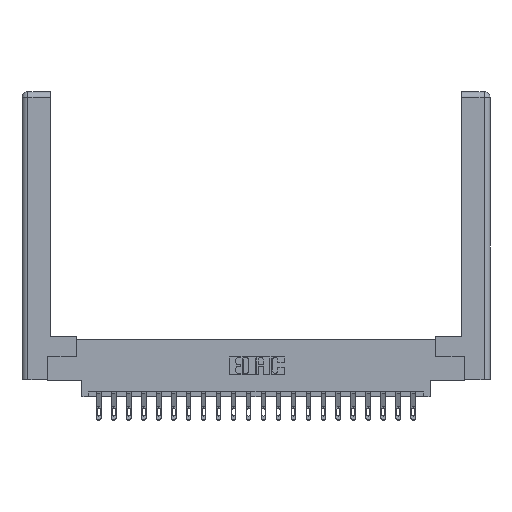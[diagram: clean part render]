
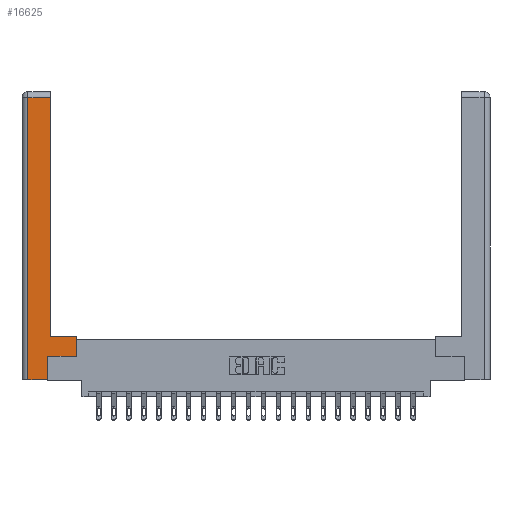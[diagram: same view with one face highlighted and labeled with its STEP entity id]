
A CAD part, top view. The second image highlights one B-rep face of the part: STEP entity #16625.
In plain terms, the highlighted planar face has unit normal (0, 0, 1).
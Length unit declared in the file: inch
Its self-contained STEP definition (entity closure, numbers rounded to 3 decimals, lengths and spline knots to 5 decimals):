
#794 = DIRECTION ( 'NONE',  ( 1., 0., 0. ) ) ;
#1180 = VERTEX_POINT ( 'NONE', #10161 ) ;
#1387 = CARTESIAN_POINT ( 'NONE',  ( 0.0615, 0., 0. ) ) ;
#1826 = VECTOR ( 'NONE', #3564, 39.37008 ) ;
#1943 = LINE ( 'NONE', #19112, #6294 ) ;
#2368 = CARTESIAN_POINT ( 'NONE',  ( 0.295, 2.94, 0. ) ) ;
#2577 = CARTESIAN_POINT ( 'NONE',  ( 0.265, 0., 0. ) ) ;
#2989 = VERTEX_POINT ( 'NONE', #10804 ) ;
#3122 = EDGE_CURVE ( 'NONE', #5500, #7006, #20719, .T. ) ;
#3294 = ORIENTED_EDGE ( 'NONE', *, *, #3122, .T. ) ;
#3403 = DIRECTION ( 'NONE',  ( 0., -1., 0. ) ) ;
#3490 = LINE ( 'NONE', #22546, #15811 ) ;
#3564 = DIRECTION ( 'NONE',  ( 1., 0., 0. ) ) ;
#3567 = CARTESIAN_POINT ( 'NONE',  ( 0., 0., 0. ) ) ;
#4233 = EDGE_CURVE ( 'NONE', #2989, #10051, #9920, .T. ) ;
#4491 = CARTESIAN_POINT ( 'NONE',  ( 0.265, 0.245, 0. ) ) ;
#4816 = LINE ( 'NONE', #18980, #5356 ) ;
#5103 = FACE_OUTER_BOUND ( 'NONE', #11005, .T. ) ;
#5356 = VECTOR ( 'NONE', #22328, 39.37008 ) ;
#5500 = VERTEX_POINT ( 'NONE', #2577 ) ;
#5528 = CARTESIAN_POINT ( 'NONE',  ( 0.565, 0.245, 0. ) ) ;
#5800 = VECTOR ( 'NONE', #9698, 39.37008 ) ;
#6276 = CARTESIAN_POINT ( 'NONE',  ( 0.565, 0.45, 0. ) ) ;
#6294 = VECTOR ( 'NONE', #3403, 39.37008 ) ;
#6546 = DIRECTION ( 'NONE',  ( -1., 0., 0. ) ) ;
#6777 = LINE ( 'NONE', #13402, #11740 ) ;
#6865 = EDGE_CURVE ( 'NONE', #11948, #5500, #20832, .T. ) ;
#7006 = VERTEX_POINT ( 'NONE', #4491 ) ;
#7509 = EDGE_CURVE ( 'NONE', #10051, #1180, #3490, .T. ) ;
#7518 = VECTOR ( 'NONE', #18393, 39.37008 ) ;
#8170 = EDGE_CURVE ( 'NONE', #1180, #8821, #4816, .T. ) ;
#8821 = VERTEX_POINT ( 'NONE', #2368 ) ;
#8831 = PLANE ( 'NONE',  #20022 ) ;
#9254 = ORIENTED_EDGE ( 'NONE', *, *, #15622, .T. ) ;
#9698 = DIRECTION ( 'NONE',  ( 0., 1., 0. ) ) ;
#9920 = LINE ( 'NONE', #11658, #5800 ) ;
#10051 = VERTEX_POINT ( 'NONE', #6276 ) ;
#10161 = CARTESIAN_POINT ( 'NONE',  ( 0.295, 0.45, 0. ) ) ;
#10804 = CARTESIAN_POINT ( 'NONE',  ( 0.565, 0.245, 0. ) ) ;
#11005 = EDGE_LOOP ( 'NONE', ( #16979, #11349, #17072, #18720, #3294, #9254, #19924, #19712 ) ) ;
#11349 = ORIENTED_EDGE ( 'NONE', *, *, #12863, .T. ) ;
#11658 = CARTESIAN_POINT ( 'NONE',  ( 0.565, 0.45, 0. ) ) ;
#11740 = VECTOR ( 'NONE', #6546, 39.37008 ) ;
#11948 = VERTEX_POINT ( 'NONE', #1387 ) ;
#12068 = VECTOR ( 'NONE', #794, 39.37008 ) ;
#12254 = DIRECTION ( 'NONE',  ( -1., 0., 0. ) ) ;
#12271 = VERTEX_POINT ( 'NONE', #17081 ) ;
#12849 = CARTESIAN_POINT ( 'NONE',  ( 0.265, 0., 0. ) ) ;
#12863 = EDGE_CURVE ( 'NONE', #8821, #12271, #6777, .T. ) ;
#13402 = CARTESIAN_POINT ( 'NONE',  ( 0.0615, 2.94, 0. ) ) ;
#15622 = EDGE_CURVE ( 'NONE', #7006, #2989, #22716, .T. ) ;
#15811 = VECTOR ( 'NONE', #12254, 39.37008 ) ;
#16625 = ADVANCED_FACE ( 'NONE', ( #5103 ), #8831, .F. ) ;
#16979 = ORIENTED_EDGE ( 'NONE', *, *, #8170, .T. ) ;
#17072 = ORIENTED_EDGE ( 'NONE', *, *, #21052, .T. ) ;
#17081 = CARTESIAN_POINT ( 'NONE',  ( 0.0615, 2.94, 0. ) ) ;
#18312 = CARTESIAN_POINT ( 'NONE',  ( 0.265, 0.245, 0. ) ) ;
#18393 = DIRECTION ( 'NONE',  ( 0., 1., 0. ) ) ;
#18720 = ORIENTED_EDGE ( 'NONE', *, *, #6865, .T. ) ;
#18980 = CARTESIAN_POINT ( 'NONE',  ( 0.295, 3., 0. ) ) ;
#19112 = CARTESIAN_POINT ( 'NONE',  ( 0.0615, 0., 0. ) ) ;
#19712 = ORIENTED_EDGE ( 'NONE', *, *, #7509, .T. ) ;
#19924 = ORIENTED_EDGE ( 'NONE', *, *, #4233, .T. ) ;
#20022 = AXIS2_PLACEMENT_3D ( 'NONE', #3567, #21144, #21068 ) ;
#20719 = LINE ( 'NONE', #18312, #7518 ) ;
#20832 = LINE ( 'NONE', #12849, #12068 ) ;
#21052 = EDGE_CURVE ( 'NONE', #12271, #11948, #1943, .T. ) ;
#21068 = DIRECTION ( 'NONE',  ( -1., 0., 0. ) ) ;
#21144 = DIRECTION ( 'NONE',  ( 0., 0., -1. ) ) ;
#22328 = DIRECTION ( 'NONE',  ( 0., 1., 0. ) ) ;
#22546 = CARTESIAN_POINT ( 'NONE',  ( 0.295, 0.45, 0. ) ) ;
#22716 = LINE ( 'NONE', #5528, #1826 ) ;
